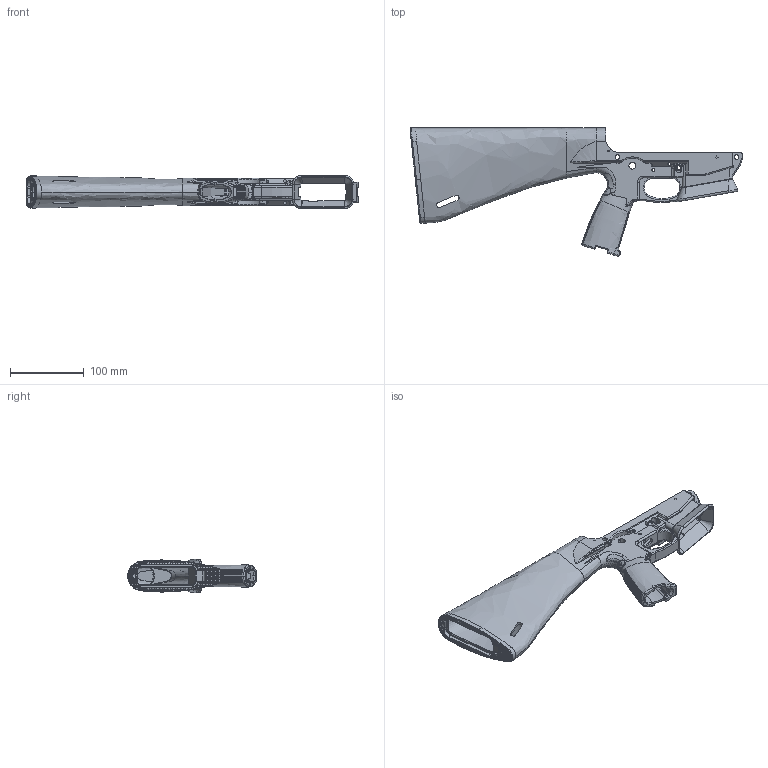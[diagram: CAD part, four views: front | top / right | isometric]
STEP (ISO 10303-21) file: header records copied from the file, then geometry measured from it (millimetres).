
FILE_DESCRIPTION (( 'STEP AP203' ), '1' );
FILE_NAME ('mbbi_monolithic.STEP', '2022-06-11T18:46:58', ( '' ), ( '' ), 'SwSTEP 2.0', 'SolidWorks 2021', '' );
FILE_SCHEMA (( 'CONFIG_CONTROL_DESIGN' ));
Products named in the file (1): mbbi_monolithic
Bounding box: 450.94 x 174.49 x 45.01 mm (x, y, z)
Volume: 467145.4 mm3; surface area: 201779.6 mm2
Topology: 1 solids, 3 shells, 3071 faces, 8598 edges, 5616 vertices
Faces by surface type: plane 2194, bspline 418, cylinder 358, torus 62, sphere 31, cone 8
Entity records: 154419 total; most frequent: CARTESIAN_POINT 87022, ORIENTED_EDGE 17138, DIRECTION 9343, EDGE_CURVE 8569, VERTEX_POINT 5612, B_SPLINE_CURVE_WITH_KNOTS 5094, AXIS2_PLACEMENT_3D 3462, EDGE_LOOP 3223
